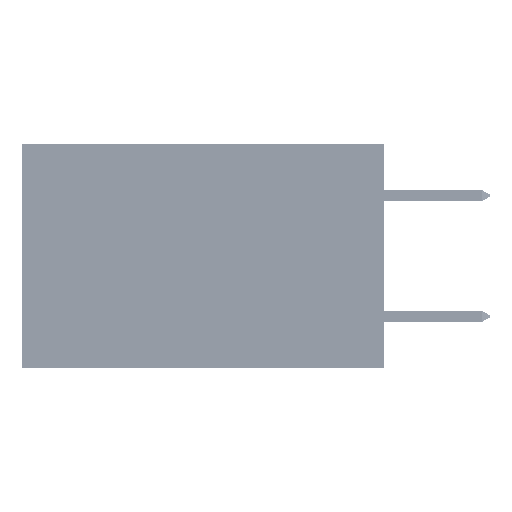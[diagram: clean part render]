
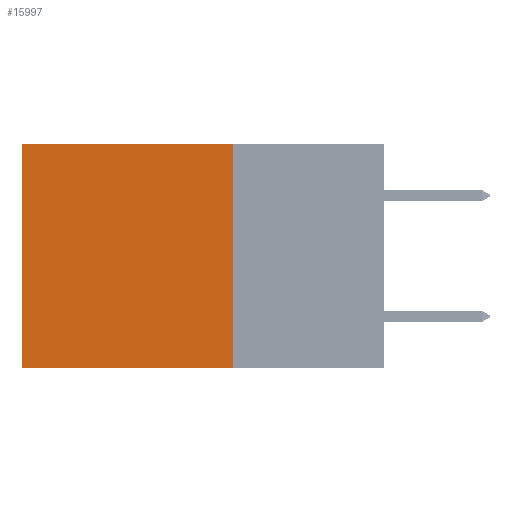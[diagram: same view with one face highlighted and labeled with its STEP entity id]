
A CAD part, left-side view. The second image highlights one B-rep face of the part: STEP entity #15997.
In plain terms, the highlighted planar face has unit normal (-1, 0, 0).
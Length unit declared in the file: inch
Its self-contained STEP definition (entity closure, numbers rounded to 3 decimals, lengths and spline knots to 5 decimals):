
#921 = LINE ( 'NONE', #23432, #14224 ) ;
#2368 = DIRECTION ( 'NONE',  ( 0., 1., 0. ) ) ;
#3097 = EDGE_CURVE ( 'NONE', #4223, #4282, #30684, .T. ) ;
#4110 = DIRECTION ( 'NONE',  ( 1., 0., 0. ) ) ;
#4223 = VERTEX_POINT ( 'NONE', #15603 ) ;
#4282 = VERTEX_POINT ( 'NONE', #26344 ) ;
#6758 = ORIENTED_EDGE ( 'NONE', *, *, #3097, .T. ) ;
#8036 = EDGE_CURVE ( 'NONE', #4282, #21652, #921, .T. ) ;
#11168 = ORIENTED_EDGE ( 'NONE', *, *, #42541, .F. ) ;
#12429 = CARTESIAN_POINT ( 'NONE',  ( 0.2875, 0.6, -0.37 ) ) ;
#14224 = VECTOR ( 'NONE', #22975, 39.37008 ) ;
#14986 = PLANE ( 'NONE',  #35652 ) ;
#15603 = CARTESIAN_POINT ( 'NONE',  ( 0.2875, 0.25, 0. ) ) ;
#15997 = ADVANCED_FACE ( 'NONE', ( #36920 ), #14986, .F. ) ;
#18329 = LINE ( 'NONE', #41154, #41190 ) ;
#21652 = VERTEX_POINT ( 'NONE', #12429 ) ;
#21657 = EDGE_CURVE ( 'NONE', #38694, #21652, #18329, .T. ) ;
#22305 = VECTOR ( 'NONE', #2368, 39.37008 ) ;
#22881 = DIRECTION ( 'NONE',  ( 0., 1., 0. ) ) ;
#22975 = DIRECTION ( 'NONE',  ( 0., 0., -1. ) ) ;
#23432 = CARTESIAN_POINT ( 'NONE',  ( 0.2875, 0.6, 0. ) ) ;
#25084 = ORIENTED_EDGE ( 'NONE', *, *, #21657, .F. ) ;
#25420 = CARTESIAN_POINT ( 'NONE',  ( 0.2875, 0.25, 0. ) ) ;
#25506 = VECTOR ( 'NONE', #26279, 39.37008 ) ;
#26279 = DIRECTION ( 'NONE',  ( 0., 0., -1. ) ) ;
#26344 = CARTESIAN_POINT ( 'NONE',  ( 0.2875, 0.6, 0. ) ) ;
#30047 = CARTESIAN_POINT ( 'NONE',  ( 0.2875, 0.25, 0. ) ) ;
#30684 = LINE ( 'NONE', #41589, #22305 ) ;
#34652 = ORIENTED_EDGE ( 'NONE', *, *, #8036, .T. ) ;
#34978 = LINE ( 'NONE', #30047, #25506 ) ;
#35652 = AXIS2_PLACEMENT_3D ( 'NONE', #25420, #4110, #39959 ) ;
#36920 = FACE_OUTER_BOUND ( 'NONE', #40911, .T. ) ;
#38694 = VERTEX_POINT ( 'NONE', #45640 ) ;
#39959 = DIRECTION ( 'NONE',  ( 0., 0., -1. ) ) ;
#40911 = EDGE_LOOP ( 'NONE', ( #34652, #25084, #11168, #6758 ) ) ;
#41154 = CARTESIAN_POINT ( 'NONE',  ( 0.2875, 0.25, -0.37 ) ) ;
#41190 = VECTOR ( 'NONE', #22881, 39.37008 ) ;
#41589 = CARTESIAN_POINT ( 'NONE',  ( 0.2875, 0.25, 0. ) ) ;
#42541 = EDGE_CURVE ( 'NONE', #4223, #38694, #34978, .T. ) ;
#45640 = CARTESIAN_POINT ( 'NONE',  ( 0.2875, 0.25, -0.37 ) ) ;
